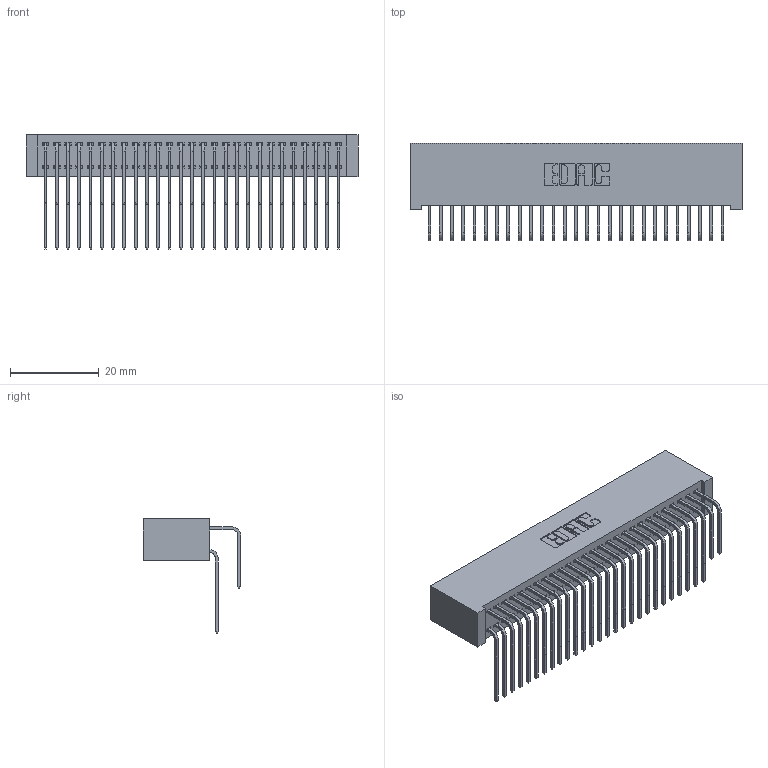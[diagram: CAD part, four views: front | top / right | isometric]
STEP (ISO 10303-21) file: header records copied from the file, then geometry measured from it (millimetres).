
FILE_DESCRIPTION (( 'STEP AP203' ), '1' );
FILE_NAME ('342-054-558-201.STEP', '2018-08-13T00:54:47', ( '' ), ( '' ), 'SwSTEP 2.0', 'SolidWorks 2016', '' );
FILE_SCHEMA (( 'CONFIG_CONTROL_DESIGN' ));
Length unit declared in the file: inch
Products named in the file (4): 342 Part_Lugless; 345-292-001_558 559 Tail - 1; 345-292-001_558 Tail - 2; 342-054-558-201
Assembly tree (55 placements, depth 2):
  342-054-558-201
    342 Part_Lugless
    345-292-001_558 559 Tail - 1  x27
    345-292-001_558 Tail - 2  x27
Bounding box: 74.83 x 21.91 x 25.78 mm (x, y, z)
Volume: 7403.3 mm3; surface area: 13536.6 mm2
Topology: 55 solids, 55 shells, 3018 faces, 8969 edges, 5906 vertices
Faces by surface type: plane 2114, cylinder 904
Entity records: 20685 total; most frequent: CARTESIAN_POINT 3493, ORIENTED_EDGE 3378, DIRECTION 2985, EDGE_CURVE 1689, VECTOR 1529, LINE 1529, VERTEX_POINT 1122, AXIS2_PLACEMENT_3D 728
